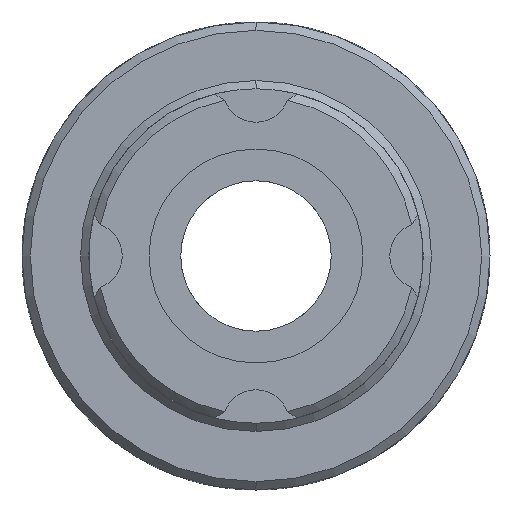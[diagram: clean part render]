
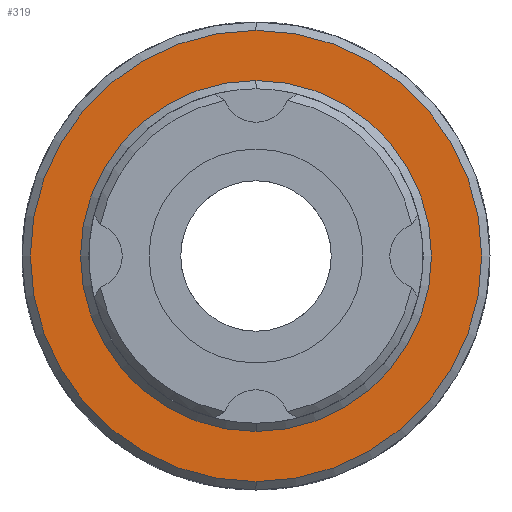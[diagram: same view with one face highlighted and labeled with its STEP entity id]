
A CAD part, left-side view. The second image highlights one B-rep face of the part: STEP entity #319.
In plain terms, the highlighted planar face has unit normal (-1, 0, 0).
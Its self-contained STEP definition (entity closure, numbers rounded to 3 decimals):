
#133 = DIRECTION ( 'NONE',  ( -1., 0., 0. ) ) ;
#136 = CARTESIAN_POINT ( 'NONE',  ( 10., 0., 0. ) ) ;
#137 = PLANE ( 'NONE',  #1101 ) ;
#139 = DIRECTION ( 'NONE',  ( 0., 0., 1. ) ) ;
#319 = ADVANCED_FACE ( 'NONE', ( #951, #953 ), #137, .T. ) ;
#423 = EDGE_CURVE ( 'NONE', #837, #882, #1461, .T. ) ;
#425 = EDGE_CURVE ( 'NONE', #847, #877, #1464, .T. ) ;
#579 = EDGE_LOOP ( 'NONE', ( #2263, #2264 ) ) ;
#586 = EDGE_LOOP ( 'NONE', ( #2265, #2266 ) ) ;
#837 = VERTEX_POINT ( 'NONE', #2081 ) ;
#847 = VERTEX_POINT ( 'NONE', #2091 ) ;
#877 = VERTEX_POINT ( 'NONE', #2121 ) ;
#882 = VERTEX_POINT ( 'NONE', #2126 ) ;
#951 = FACE_OUTER_BOUND ( 'NONE', #579, .T. ) ;
#953 = FACE_BOUND ( 'NONE', #586, .T. ) ;
#1076 = EDGE_CURVE ( 'NONE', #877, #847, #1547, .T. ) ;
#1077 = EDGE_CURVE ( 'NONE', #882, #837, #1565, .T. ) ;
#1101 = AXIS2_PLACEMENT_3D ( 'NONE', #136, #133, #139 ) ;
#1342 = CARTESIAN_POINT ( 'NONE',  ( 10., 0., 0. ) ) ;
#1343 = DIRECTION ( 'NONE',  ( 1., 0., 0. ) ) ;
#1344 = DIRECTION ( 'NONE',  ( 0., 0., 1. ) ) ;
#1347 = CARTESIAN_POINT ( 'NONE',  ( 10., 0., 0. ) ) ;
#1348 = DIRECTION ( 'NONE',  ( -1., 0., 0. ) ) ;
#1349 = DIRECTION ( 'NONE',  ( 0., 0., 1. ) ) ;
#1409 = AXIS2_PLACEMENT_3D ( 'NONE', #1342, #1343, #1344 ) ;
#1410 = AXIS2_PLACEMENT_3D ( 'NONE', #1347, #1348, #1349 ) ;
#1443 = AXIS2_PLACEMENT_3D ( 'NONE', #2176, #2177, #2178 ) ;
#1444 = AXIS2_PLACEMENT_3D ( 'NONE', #2180, #2181, #2182 ) ;
#1461 = CIRCLE ( 'NONE', #1409, 10.5 ) ;
#1464 = CIRCLE ( 'NONE', #1410, 13.5 ) ;
#1547 = CIRCLE ( 'NONE', #1443, 13.5 ) ;
#1565 = CIRCLE ( 'NONE', #1444, 10.5 ) ;
#2081 = CARTESIAN_POINT ( 'NONE',  ( 10., 0., -10.5 ) ) ;
#2091 = CARTESIAN_POINT ( 'NONE',  ( 10., 0., 13.5 ) ) ;
#2121 = CARTESIAN_POINT ( 'NONE',  ( 10., 0., -13.5 ) ) ;
#2126 = CARTESIAN_POINT ( 'NONE',  ( 10., 0., 10.5 ) ) ;
#2176 = CARTESIAN_POINT ( 'NONE',  ( 10., 0., 0. ) ) ;
#2177 = DIRECTION ( 'NONE',  ( -1., 0., 0. ) ) ;
#2178 = DIRECTION ( 'NONE',  ( 0., 0., 1. ) ) ;
#2180 = CARTESIAN_POINT ( 'NONE',  ( 10., 0., 0. ) ) ;
#2181 = DIRECTION ( 'NONE',  ( 1., 0., 0. ) ) ;
#2182 = DIRECTION ( 'NONE',  ( 0., 0., 1. ) ) ;
#2263 = ORIENTED_EDGE ( 'NONE', *, *, #1076, .T. ) ;
#2264 = ORIENTED_EDGE ( 'NONE', *, *, #425, .T. ) ;
#2265 = ORIENTED_EDGE ( 'NONE', *, *, #423, .T. ) ;
#2266 = ORIENTED_EDGE ( 'NONE', *, *, #1077, .T. ) ;
